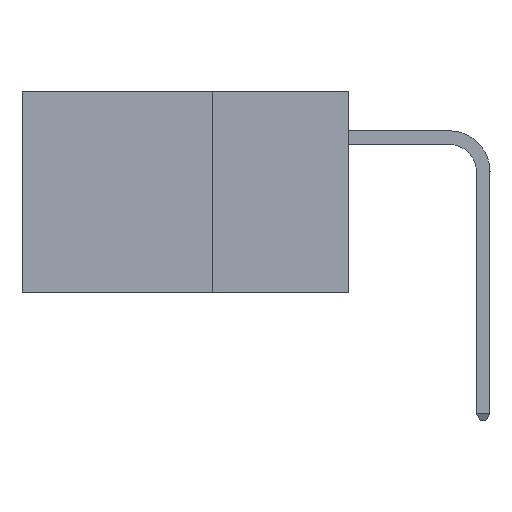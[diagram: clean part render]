
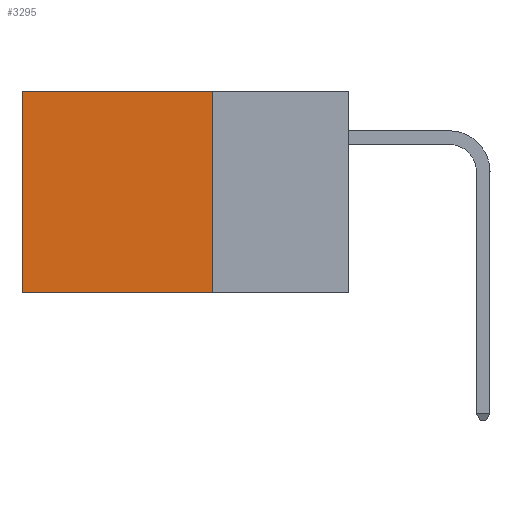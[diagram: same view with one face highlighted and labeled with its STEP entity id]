
A CAD part, left-side view. The second image highlights one B-rep face of the part: STEP entity #3295.
In plain terms, the highlighted planar face has unit normal (-1, 0, 0).
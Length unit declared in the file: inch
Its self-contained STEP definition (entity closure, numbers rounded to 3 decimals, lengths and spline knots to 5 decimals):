
#675 = ORIENTED_EDGE ( 'NONE', *, *, #16223, .T. ) ;
#688 = ORIENTED_EDGE ( 'NONE', *, *, #10851, .F. ) ;
#886 = CARTESIAN_POINT ( 'NONE',  ( 0.2875, 0.25, 0. ) ) ;
#1109 = DIRECTION ( 'NONE',  ( 1., 0., 0. ) ) ;
#1663 = CARTESIAN_POINT ( 'NONE',  ( 0.2875, 0.25, 0. ) ) ;
#1778 = LINE ( 'NONE', #15437, #9474 ) ;
#1973 = VERTEX_POINT ( 'NONE', #16060 ) ;
#2734 = CARTESIAN_POINT ( 'NONE',  ( 0.2875, 0.6, -0.37 ) ) ;
#2925 = AXIS2_PLACEMENT_3D ( 'NONE', #886, #1109, #18010 ) ;
#3295 = ADVANCED_FACE ( 'NONE', ( #4485 ), #10294, .F. ) ;
#4485 = FACE_OUTER_BOUND ( 'NONE', #6057, .T. ) ;
#4540 = LINE ( 'NONE', #1663, #12669 ) ;
#4943 = DIRECTION ( 'NONE',  ( 0., 1., 0. ) ) ;
#6057 = EDGE_LOOP ( 'NONE', ( #16472, #688, #9826, #675 ) ) ;
#6734 = CARTESIAN_POINT ( 'NONE',  ( 0.2875, 0.25, 0. ) ) ;
#6787 = CARTESIAN_POINT ( 'NONE',  ( 0.2875, 0.25, -0.37 ) ) ;
#8797 = VECTOR ( 'NONE', #11374, 39.37008 ) ;
#8936 = EDGE_CURVE ( 'NONE', #1973, #14704, #21198, .T. ) ;
#9251 = VECTOR ( 'NONE', #16452, 39.37008 ) ;
#9474 = VECTOR ( 'NONE', #10663, 39.37008 ) ;
#9757 = CARTESIAN_POINT ( 'NONE',  ( 0.2875, 0.6, 0. ) ) ;
#9826 = ORIENTED_EDGE ( 'NONE', *, *, #13425, .F. ) ;
#10294 = PLANE ( 'NONE',  #2925 ) ;
#10663 = DIRECTION ( 'NONE',  ( 0., 0., -1. ) ) ;
#10851 = EDGE_CURVE ( 'NONE', #15718, #14704, #18875, .T. ) ;
#11374 = DIRECTION ( 'NONE',  ( 0., 0., -1. ) ) ;
#12669 = VECTOR ( 'NONE', #4943, 39.37008 ) ;
#13425 = EDGE_CURVE ( 'NONE', #20681, #15718, #1778, .T. ) ;
#13459 = CARTESIAN_POINT ( 'NONE',  ( 0.2875, 0.25, -0.37 ) ) ;
#14704 = VERTEX_POINT ( 'NONE', #2734 ) ;
#15437 = CARTESIAN_POINT ( 'NONE',  ( 0.2875, 0.25, 0. ) ) ;
#15718 = VERTEX_POINT ( 'NONE', #13459 ) ;
#16060 = CARTESIAN_POINT ( 'NONE',  ( 0.2875, 0.6, 0. ) ) ;
#16223 = EDGE_CURVE ( 'NONE', #20681, #1973, #4540, .T. ) ;
#16452 = DIRECTION ( 'NONE',  ( 0., 1., 0. ) ) ;
#16472 = ORIENTED_EDGE ( 'NONE', *, *, #8936, .T. ) ;
#18010 = DIRECTION ( 'NONE',  ( 0., 0., -1. ) ) ;
#18875 = LINE ( 'NONE', #6787, #9251 ) ;
#20681 = VERTEX_POINT ( 'NONE', #6734 ) ;
#21198 = LINE ( 'NONE', #9757, #8797 ) ;
